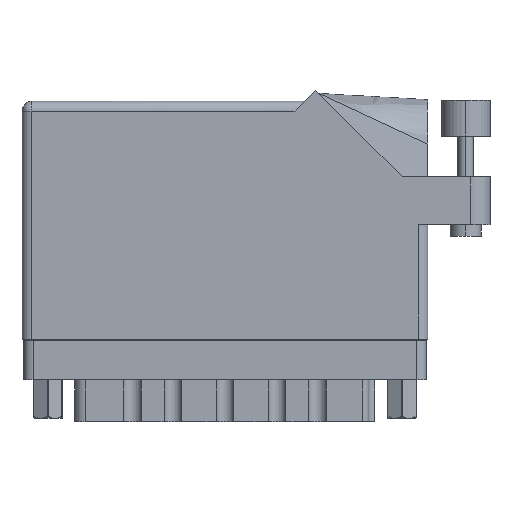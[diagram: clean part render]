
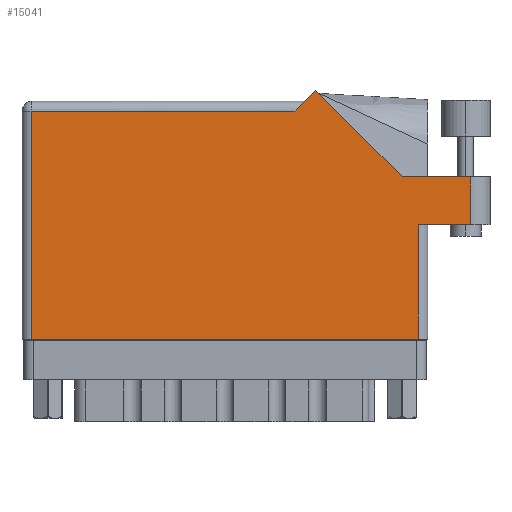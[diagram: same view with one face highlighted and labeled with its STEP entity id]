
A CAD part, front view. The second image highlights one B-rep face of the part: STEP entity #15041.
In plain terms, the highlighted face is planar.
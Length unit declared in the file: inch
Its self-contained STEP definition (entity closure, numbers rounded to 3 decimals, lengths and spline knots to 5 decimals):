
#818 = LINE ( 'NONE', #6763, #59469 ) ;
#841 = VERTEX_POINT ( 'NONE', #51821 ) ;
#2199 = CARTESIAN_POINT ( 'NONE',  ( 0.062, 0., 0. ) ) ;
#2627 = CARTESIAN_POINT ( 'NONE',  ( 2.887, 1.044, 0. ) ) ;
#3581 = LINE ( 'NONE', #2199, #12613 ) ;
#3742 = EDGE_CURVE ( 'NONE', #18651, #6093, #3581, .T. ) ;
#4623 = ORIENTED_EDGE ( 'NONE', *, *, #37865, .T. ) ;
#5160 = LINE ( 'NONE', #2627, #37443 ) ;
#6093 = VERTEX_POINT ( 'NONE', #59255 ) ;
#6763 = CARTESIAN_POINT ( 'NONE',  ( 3.012, 1.044, 0. ) ) ;
#8515 = DIRECTION ( 'NONE',  ( -0.707, -0.707, 0. ) ) ;
#8613 = DIRECTION ( 'NONE',  ( -1., 0., 0. ) ) ;
#8676 = VECTOR ( 'NONE', #48055, 39.37008 ) ;
#10923 = ORIENTED_EDGE ( 'NONE', *, *, #53302, .T. ) ;
#11608 = DIRECTION ( 'NONE',  ( -1., 0., 0. ) ) ;
#11729 = VECTOR ( 'NONE', #8515, 39.37008 ) ;
#12613 = VECTOR ( 'NONE', #50125, 39.37008 ) ;
#12925 = ORIENTED_EDGE ( 'NONE', *, *, #50952, .T. ) ;
#13159 = VERTEX_POINT ( 'NONE', #27659 ) ;
#13338 = ORIENTED_EDGE ( 'NONE', *, *, #3742, .T. ) ;
#14494 = FACE_OUTER_BOUND ( 'NONE', #47001, .T. ) ;
#15041 = ADVANCED_FACE ( 'NONE', ( #14494 ), #50958, .F. ) ;
#16072 = VECTOR ( 'NONE', #21259, 39.37008 ) ;
#17019 = DIRECTION ( 'NONE',  ( 0., 1., 0. ) ) ;
#17552 = DIRECTION ( 'NONE',  ( -1., 0., 0. ) ) ;
#17650 = EDGE_CURVE ( 'NONE', #51349, #53416, #19817, .T. ) ;
#18651 = VERTEX_POINT ( 'NONE', #37481 ) ;
#19817 = LINE ( 'NONE', #59273, #16072 ) ;
#21259 = DIRECTION ( 'NONE',  ( 1., 0., 0. ) ) ;
#22473 = EDGE_CURVE ( 'NONE', #46345, #51349, #42488, .T. ) ;
#26292 = LINE ( 'NONE', #31886, #38378 ) ;
#26609 = EDGE_CURVE ( 'NONE', #43803, #45855, #818, .T. ) ;
#26676 = VECTOR ( 'NONE', #17019, 39.37008 ) ;
#26945 = DIRECTION ( 'NONE',  ( 0., 1., 0. ) ) ;
#27659 = CARTESIAN_POINT ( 'NONE',  ( 1.88971, 1.60071, 0. ) ) ;
#28000 = CARTESIAN_POINT ( 'NONE',  ( 0., 0., 0. ) ) ;
#29541 = EDGE_CURVE ( 'NONE', #53416, #43803, #5160, .T. ) ;
#29684 = CARTESIAN_POINT ( 'NONE',  ( 2.55, 0., 0. ) ) ;
#31432 = CARTESIAN_POINT ( 'NONE',  ( 2.55, 0.737, 0. ) ) ;
#31886 = CARTESIAN_POINT ( 'NONE',  ( 0., 1.468, 0. ) ) ;
#32398 = DIRECTION ( 'NONE',  ( 0., 0., -1. ) ) ;
#33396 = ORIENTED_EDGE ( 'NONE', *, *, #26609, .T. ) ;
#33941 = CARTESIAN_POINT ( 'NONE',  ( 2.44642, 1.044, 0. ) ) ;
#35326 = CARTESIAN_POINT ( 'NONE',  ( 2.44642, 1.044, 0. ) ) ;
#37267 = CARTESIAN_POINT ( 'NONE',  ( 0., 1.53, 0. ) ) ;
#37443 = VECTOR ( 'NONE', #26945, 39.37008 ) ;
#37481 = CARTESIAN_POINT ( 'NONE',  ( 0.062, 1.468, 0. ) ) ;
#37708 = DIRECTION ( 'NONE',  ( 1., 0., 0. ) ) ;
#37865 = EDGE_CURVE ( 'NONE', #841, #18651, #26292, .T. ) ;
#38378 = VECTOR ( 'NONE', #8613, 39.37008 ) ;
#41838 = CARTESIAN_POINT ( 'NONE',  ( 2.55, 0.737, 0. ) ) ;
#42488 = LINE ( 'NONE', #31432, #26676 ) ;
#42792 = LINE ( 'NONE', #28000, #52574 ) ;
#43803 = VERTEX_POINT ( 'NONE', #44613 ) ;
#43898 = ORIENTED_EDGE ( 'NONE', *, *, #29541, .T. ) ;
#44613 = CARTESIAN_POINT ( 'NONE',  ( 2.887, 1.044, 0. ) ) ;
#45855 = VERTEX_POINT ( 'NONE', #35326 ) ;
#45989 = AXIS2_PLACEMENT_3D ( 'NONE', #37267, #32398, #17552 ) ;
#46345 = VERTEX_POINT ( 'NONE', #29684 ) ;
#46722 = CARTESIAN_POINT ( 'NONE',  ( 1.819, 1.53, 0. ) ) ;
#47001 = EDGE_LOOP ( 'NONE', ( #61122, #43898, #33396, #60452, #10923, #4623, #13338, #12925, #49221 ) ) ;
#48055 = DIRECTION ( 'NONE',  ( -0.707, 0.707, 0. ) ) ;
#48201 = CARTESIAN_POINT ( 'NONE',  ( 2.887, 0.737, 0. ) ) ;
#49221 = ORIENTED_EDGE ( 'NONE', *, *, #22473, .T. ) ;
#50125 = DIRECTION ( 'NONE',  ( 0., -1., 0. ) ) ;
#50952 = EDGE_CURVE ( 'NONE', #6093, #46345, #42792, .T. ) ;
#50958 = PLANE ( 'NONE',  #45989 ) ;
#51349 = VERTEX_POINT ( 'NONE', #41838 ) ;
#51821 = CARTESIAN_POINT ( 'NONE',  ( 1.757, 1.468, 0. ) ) ;
#52574 = VECTOR ( 'NONE', #37708, 39.37008 ) ;
#53302 = EDGE_CURVE ( 'NONE', #13159, #841, #54592, .T. ) ;
#53416 = VERTEX_POINT ( 'NONE', #48201 ) ;
#54592 = LINE ( 'NONE', #46722, #11729 ) ;
#58286 = LINE ( 'NONE', #33941, #8676 ) ;
#59255 = CARTESIAN_POINT ( 'NONE',  ( 0.062, 0., 0. ) ) ;
#59273 = CARTESIAN_POINT ( 'NONE',  ( 2.612, 0.737, 0. ) ) ;
#59469 = VECTOR ( 'NONE', #11608, 39.37008 ) ;
#59981 = EDGE_CURVE ( 'NONE', #45855, #13159, #58286, .T. ) ;
#60452 = ORIENTED_EDGE ( 'NONE', *, *, #59981, .T. ) ;
#61122 = ORIENTED_EDGE ( 'NONE', *, *, #17650, .T. ) ;
